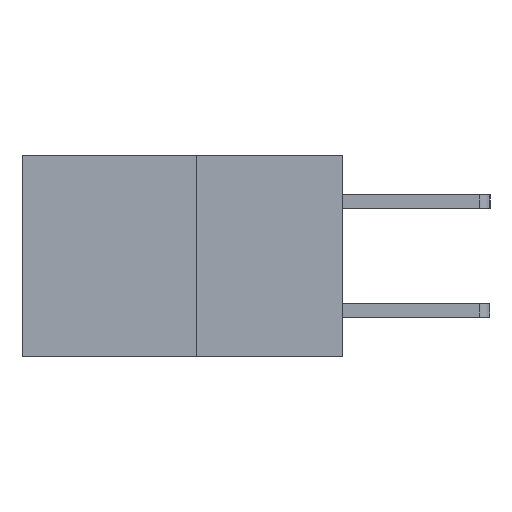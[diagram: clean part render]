
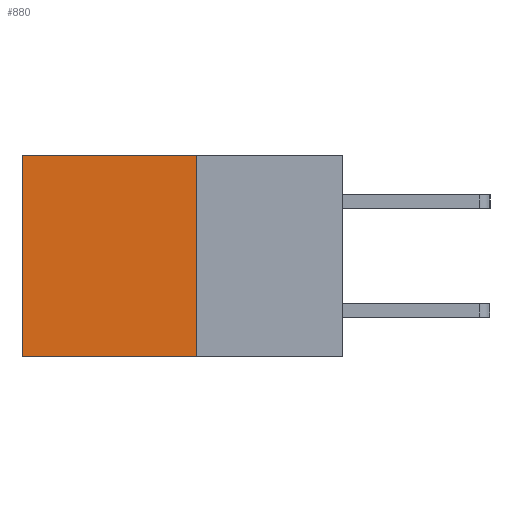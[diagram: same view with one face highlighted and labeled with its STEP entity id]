
A CAD part, left-side view. The second image highlights one B-rep face of the part: STEP entity #880.
In plain terms, the highlighted planar face has unit normal (-1, 0, 0).
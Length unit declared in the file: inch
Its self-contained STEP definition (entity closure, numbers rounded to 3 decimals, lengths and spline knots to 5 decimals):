
#11 = DIRECTION ( 'NONE',  ( 0., 0., -1. ) ) ;
#125 = CARTESIAN_POINT ( 'NONE',  ( 0.277, 0.59, -0.37 ) ) ;
#245 = DIRECTION ( 'NONE',  ( 0., 0., -1. ) ) ;
#817 = VECTOR ( 'NONE', #11, 39.37008 ) ;
#880 = ADVANCED_FACE ( 'NONE', ( #1574 ), #2409, .F. ) ;
#886 = LINE ( 'NONE', #4724, #4891 ) ;
#940 = DIRECTION ( 'NONE',  ( 1., 0., 0. ) ) ;
#1546 = EDGE_CURVE ( 'NONE', #3312, #6439, #7011, .T. ) ;
#1574 = FACE_OUTER_BOUND ( 'NONE', #5660, .T. ) ;
#1806 = CARTESIAN_POINT ( 'NONE',  ( 0.277, 0.27, 0. ) ) ;
#2409 = PLANE ( 'NONE',  #7137 ) ;
#2423 = LINE ( 'NONE', #5246, #2681 ) ;
#2447 = EDGE_CURVE ( 'NONE', #3297, #3312, #2423, .T. ) ;
#2451 = CARTESIAN_POINT ( 'NONE',  ( 0.277, 0.27, -0.37 ) ) ;
#2681 = VECTOR ( 'NONE', #5462, 39.37008 ) ;
#3070 = VERTEX_POINT ( 'NONE', #2451 ) ;
#3297 = VERTEX_POINT ( 'NONE', #1806 ) ;
#3312 = VERTEX_POINT ( 'NONE', #3481 ) ;
#3481 = CARTESIAN_POINT ( 'NONE',  ( 0.277, 0.59, 0. ) ) ;
#3992 = DIRECTION ( 'NONE',  ( 0., 0., -1. ) ) ;
#4402 = EDGE_CURVE ( 'NONE', #3070, #6439, #5110, .T. ) ;
#4724 = CARTESIAN_POINT ( 'NONE',  ( 0.277, 0.27, -0.37 ) ) ;
#4891 = VECTOR ( 'NONE', #3992, 39.37008 ) ;
#5110 = LINE ( 'NONE', #6482, #8761 ) ;
#5246 = CARTESIAN_POINT ( 'NONE',  ( 0.277, 0.27, 0. ) ) ;
#5462 = DIRECTION ( 'NONE',  ( 0., 1., 0. ) ) ;
#5660 = EDGE_LOOP ( 'NONE', ( #6761, #6841, #6873, #6881 ) ) ;
#6005 = CARTESIAN_POINT ( 'NONE',  ( 0.277, 0.59, -0.37 ) ) ;
#6439 = VERTEX_POINT ( 'NONE', #6005 ) ;
#6482 = CARTESIAN_POINT ( 'NONE',  ( 0.277, 0.27, -0.37 ) ) ;
#6761 = ORIENTED_EDGE ( 'NONE', *, *, #1546, .T. ) ;
#6841 = ORIENTED_EDGE ( 'NONE', *, *, #4402, .F. ) ;
#6873 = ORIENTED_EDGE ( 'NONE', *, *, #8432, .F. ) ;
#6881 = ORIENTED_EDGE ( 'NONE', *, *, #2447, .T. ) ;
#7011 = LINE ( 'NONE', #125, #817 ) ;
#7137 = AXIS2_PLACEMENT_3D ( 'NONE', #9068, #940, #245 ) ;
#7215 = DIRECTION ( 'NONE',  ( 0., 1., 0. ) ) ;
#8432 = EDGE_CURVE ( 'NONE', #3297, #3070, #886, .T. ) ;
#8761 = VECTOR ( 'NONE', #7215, 39.37008 ) ;
#9068 = CARTESIAN_POINT ( 'NONE',  ( 0.277, 0.27, -0.37 ) ) ;
